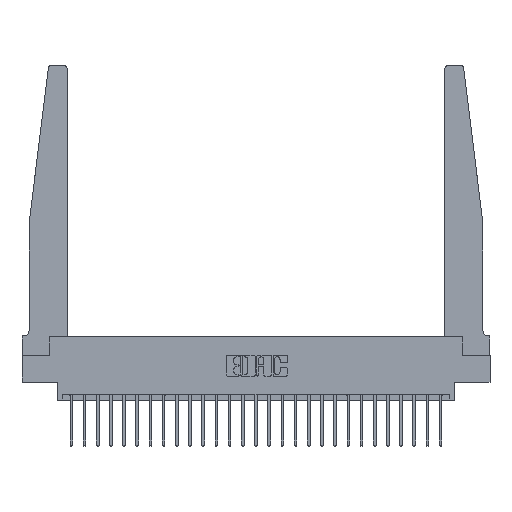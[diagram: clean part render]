
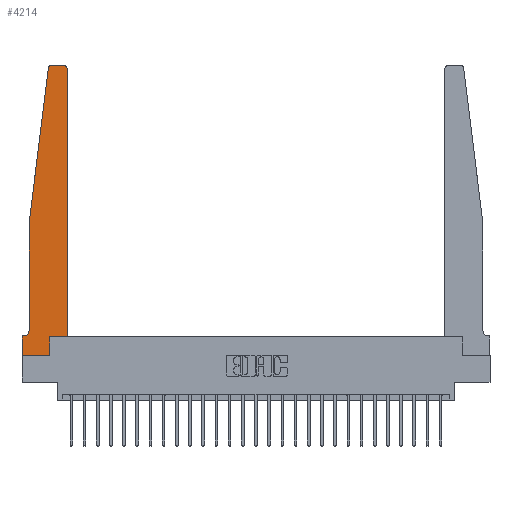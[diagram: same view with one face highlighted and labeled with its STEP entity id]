
A CAD part, top view. The second image highlights one B-rep face of the part: STEP entity #4214.
In plain terms, the highlighted planar face has unit normal (0, 0, 1).
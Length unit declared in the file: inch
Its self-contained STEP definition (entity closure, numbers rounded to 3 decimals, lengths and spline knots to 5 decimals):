
#243 = VERTEX_POINT ( 'NONE', #15301 ) ;
#253 = VECTOR ( 'NONE', #4110, 39.37008 ) ;
#643 = DIRECTION ( 'NONE',  ( 0., 1., 0. ) ) ;
#967 = DIRECTION ( 'NONE',  ( -0.122, -0.992, 0. ) ) ;
#1580 = CARTESIAN_POINT ( 'NONE',  ( 0., 0., 0.37 ) ) ;
#1728 = VERTEX_POINT ( 'NONE', #2740 ) ;
#2059 = CARTESIAN_POINT ( 'NONE',  ( 0.065, 1.25, 0.37 ) ) ;
#2147 = LINE ( 'NONE', #11262, #22566 ) ;
#2222 = VECTOR ( 'NONE', #12136, 39.37008 ) ;
#2253 = CARTESIAN_POINT ( 'NONE',  ( 0.425, 2.72, 0.37 ) ) ;
#2461 = EDGE_CURVE ( 'NONE', #22050, #3344, #19755, .T. ) ;
#2505 = LINE ( 'NONE', #3364, #17742 ) ;
#2617 = ORIENTED_EDGE ( 'NONE', *, *, #14925, .T. ) ;
#2740 = CARTESIAN_POINT ( 'NONE',  ( 0.425, 0.18, 0.37 ) ) ;
#2760 = ORIENTED_EDGE ( 'NONE', *, *, #13868, .T. ) ;
#2795 = PLANE ( 'NONE',  #16481 ) ;
#3199 = EDGE_CURVE ( 'NONE', #18377, #22050, #14878, .T. ) ;
#3344 = VERTEX_POINT ( 'NONE', #18030 ) ;
#3364 = CARTESIAN_POINT ( 'NONE',  ( 0.425, 0.18, 0.37 ) ) ;
#4032 = DIRECTION ( 'NONE',  ( 0., 1., 0. ) ) ;
#4109 = ORIENTED_EDGE ( 'NONE', *, *, #15435, .T. ) ;
#4110 = DIRECTION ( 'NONE',  ( 0., -1., 0. ) ) ;
#4214 = ADVANCED_FACE ( 'NONE', ( #9499 ), #2795, .T. ) ;
#5293 = DIRECTION ( 'NONE',  ( -1., 0., 0. ) ) ;
#5371 = DIRECTION ( 'NONE',  ( 1., 0., 0. ) ) ;
#5448 = VERTEX_POINT ( 'NONE', #24409 ) ;
#5916 = ORIENTED_EDGE ( 'NONE', *, *, #7341, .T. ) ;
#6817 = DIRECTION ( 'NONE',  ( 0., 0., 1. ) ) ;
#7046 = VECTOR ( 'NONE', #643, 39.37008 ) ;
#7074 = CARTESIAN_POINT ( 'NONE',  ( 0.065, 0.1875, 0.37 ) ) ;
#7223 = VERTEX_POINT ( 'NONE', #14201 ) ;
#7341 = EDGE_CURVE ( 'NONE', #5448, #16035, #24000, .T. ) ;
#7652 = VERTEX_POINT ( 'NONE', #1580 ) ;
#8019 = CARTESIAN_POINT ( 'NONE',  ( 0.425, 0.18, 0.37 ) ) ;
#8282 = VERTEX_POINT ( 'NONE', #13174 ) ;
#8714 = DIRECTION ( 'NONE',  ( 0., 0., 1. ) ) ;
#9499 = FACE_OUTER_BOUND ( 'NONE', #20224, .T. ) ;
#9669 = VECTOR ( 'NONE', #4032, 39.37008 ) ;
#9726 = CARTESIAN_POINT ( 'NONE',  ( 0.015, 0.2375, 0.37 ) ) ;
#9818 = AXIS2_PLACEMENT_3D ( 'NONE', #20528, #8714, #22491 ) ;
#9854 = DIRECTION ( 'NONE',  ( 0., 0., 1. ) ) ;
#10284 = LINE ( 'NONE', #8019, #9669 ) ;
#10768 = AXIS2_PLACEMENT_3D ( 'NONE', #9726, #23497, #11708 ) ;
#10894 = LINE ( 'NONE', #2059, #253 ) ;
#10951 = ORIENTED_EDGE ( 'NONE', *, *, #25308, .T. ) ;
#11262 = CARTESIAN_POINT ( 'NONE',  ( 0.25, 2.75, 0.37 ) ) ;
#11461 = LINE ( 'NONE', #16948, #20695 ) ;
#11675 = ORIENTED_EDGE ( 'NONE', *, *, #2461, .T. ) ;
#11708 = DIRECTION ( 'NONE',  ( -1., 0., 0. ) ) ;
#12136 = DIRECTION ( 'NONE',  ( 1., 0., 0. ) ) ;
#12236 = CARTESIAN_POINT ( 'NONE',  ( 0., 0., 0.37 ) ) ;
#12483 = LINE ( 'NONE', #17956, #22326 ) ;
#12705 = ORIENTED_EDGE ( 'NONE', *, *, #18503, .T. ) ;
#12822 = LINE ( 'NONE', #12236, #2222 ) ;
#13174 = CARTESIAN_POINT ( 'NONE',  ( 0.27653, 2.75, 0.37 ) ) ;
#13227 = CIRCLE ( 'NONE', #22075, 0.03 ) ;
#13868 = EDGE_CURVE ( 'NONE', #7652, #5448, #12822, .T. ) ;
#14201 = CARTESIAN_POINT ( 'NONE',  ( 0.395, 2.75, 0.37 ) ) ;
#14621 = CARTESIAN_POINT ( 'NONE',  ( 0.2605, 0.18, 0.37 ) ) ;
#14878 = CIRCLE ( 'NONE', #10768, 0.05 ) ;
#14925 = EDGE_CURVE ( 'NONE', #1728, #23927, #10284, .T. ) ;
#14997 = ORIENTED_EDGE ( 'NONE', *, *, #3199, .T. ) ;
#15037 = EDGE_CURVE ( 'NONE', #8282, #243, #22899, .T. ) ;
#15301 = CARTESIAN_POINT ( 'NONE',  ( 0.24675, 2.72367, 0.37 ) ) ;
#15435 = EDGE_CURVE ( 'NONE', #15505, #18377, #10894, .T. ) ;
#15493 = ORIENTED_EDGE ( 'NONE', *, *, #22418, .T. ) ;
#15505 = VERTEX_POINT ( 'NONE', #24029 ) ;
#15670 = ORIENTED_EDGE ( 'NONE', *, *, #15037, .T. ) ;
#16035 = VERTEX_POINT ( 'NONE', #17623 ) ;
#16481 = AXIS2_PLACEMENT_3D ( 'NONE', #18667, #6817, #20617 ) ;
#16948 = CARTESIAN_POINT ( 'NONE',  ( 0.065, 1.25, 0.37 ) ) ;
#17623 = CARTESIAN_POINT ( 'NONE',  ( 0.2605, 0.18, 0.37 ) ) ;
#17742 = VECTOR ( 'NONE', #5371, 39.37008 ) ;
#17956 = CARTESIAN_POINT ( 'NONE',  ( 0., 0., 0.37 ) ) ;
#18030 = CARTESIAN_POINT ( 'NONE',  ( 0., 0.1875, 0.37 ) ) ;
#18377 = VERTEX_POINT ( 'NONE', #25083 ) ;
#18503 = EDGE_CURVE ( 'NONE', #23927, #7223, #13227, .T. ) ;
#18667 = CARTESIAN_POINT ( 'NONE',  ( 0., 0.1875, 0.37 ) ) ;
#18936 = DIRECTION ( 'NONE',  ( -1., 0., 0. ) ) ;
#19177 = VECTOR ( 'NONE', #18936, 39.37008 ) ;
#19755 = LINE ( 'NONE', #7074, #19177 ) ;
#19906 = DIRECTION ( 'NONE',  ( 0., -1., 0. ) ) ;
#20224 = EDGE_LOOP ( 'NONE', ( #24083, #15670, #10951, #4109, #14997, #11675, #15493, #2760, #5916, #23870, #2617, #12705 ) ) ;
#20528 = CARTESIAN_POINT ( 'NONE',  ( 0.27653, 2.72, 0.37 ) ) ;
#20617 = DIRECTION ( 'NONE',  ( 1., 0., 0. ) ) ;
#20695 = VECTOR ( 'NONE', #967, 39.37008 ) ;
#21645 = CARTESIAN_POINT ( 'NONE',  ( 0.395, 2.72, 0.37 ) ) ;
#22050 = VERTEX_POINT ( 'NONE', #22651 ) ;
#22075 = AXIS2_PLACEMENT_3D ( 'NONE', #21645, #9854, #23620 ) ;
#22326 = VECTOR ( 'NONE', #19906, 39.37008 ) ;
#22418 = EDGE_CURVE ( 'NONE', #3344, #7652, #12483, .T. ) ;
#22491 = DIRECTION ( 'NONE',  ( 1., 0., 0. ) ) ;
#22566 = VECTOR ( 'NONE', #5293, 39.37008 ) ;
#22651 = CARTESIAN_POINT ( 'NONE',  ( 0.015, 0.1875, 0.37 ) ) ;
#22899 = CIRCLE ( 'NONE', #9818, 0.03 ) ;
#23497 = DIRECTION ( 'NONE',  ( 0., 0., -1. ) ) ;
#23542 = EDGE_CURVE ( 'NONE', #7223, #8282, #2147, .T. ) ;
#23620 = DIRECTION ( 'NONE',  ( 1., 0., 0. ) ) ;
#23870 = ORIENTED_EDGE ( 'NONE', *, *, #25424, .T. ) ;
#23927 = VERTEX_POINT ( 'NONE', #2253 ) ;
#24000 = LINE ( 'NONE', #14621, #7046 ) ;
#24029 = CARTESIAN_POINT ( 'NONE',  ( 0.065, 1.25, 0.37 ) ) ;
#24083 = ORIENTED_EDGE ( 'NONE', *, *, #23542, .T. ) ;
#24409 = CARTESIAN_POINT ( 'NONE',  ( 0.2605, 0., 0.37 ) ) ;
#25083 = CARTESIAN_POINT ( 'NONE',  ( 0.065, 0.2375, 0.37 ) ) ;
#25308 = EDGE_CURVE ( 'NONE', #243, #15505, #11461, .T. ) ;
#25424 = EDGE_CURVE ( 'NONE', #16035, #1728, #2505, .T. ) ;
